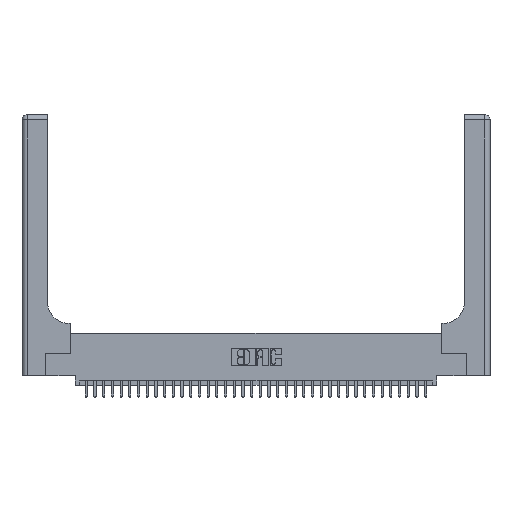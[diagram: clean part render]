
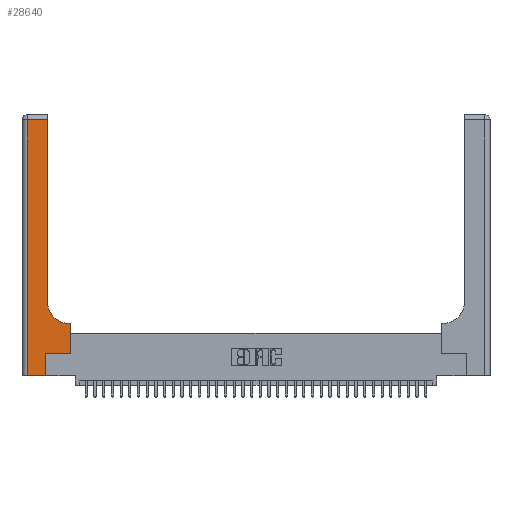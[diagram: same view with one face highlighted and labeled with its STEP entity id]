
A CAD part, top view. The second image highlights one B-rep face of the part: STEP entity #28640.
In plain terms, the highlighted planar face has unit normal (0, 0, 1).
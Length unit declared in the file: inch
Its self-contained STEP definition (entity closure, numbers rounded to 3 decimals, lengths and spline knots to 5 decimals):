
#216 = LINE ( 'NONE', #23032, #2450 ) ;
#758 = VERTEX_POINT ( 'NONE', #33562 ) ;
#1749 = ORIENTED_EDGE ( 'NONE', *, *, #3588, .T. ) ;
#1945 = FACE_OUTER_BOUND ( 'NONE', #30530, .T. ) ;
#2450 = VECTOR ( 'NONE', #5785, 39.37008 ) ;
#3264 = VERTEX_POINT ( 'NONE', #5364 ) ;
#3588 = EDGE_CURVE ( 'NONE', #25529, #7058, #6715, .T. ) ;
#4410 = VERTEX_POINT ( 'NONE', #25109 ) ;
#4511 = CARTESIAN_POINT ( 'NONE',  ( 0.269, 0.25, 0.37 ) ) ;
#5068 = VECTOR ( 'NONE', #15539, 39.37008 ) ;
#5190 = EDGE_CURVE ( 'NONE', #35783, #10188, #32566, .T. ) ;
#5364 = CARTESIAN_POINT ( 'NONE',  ( 0.269, 0., 0.37 ) ) ;
#5785 = DIRECTION ( 'NONE',  ( 1., 0., 0. ) ) ;
#5846 = EDGE_CURVE ( 'NONE', #9022, #7804, #28762, .T. ) ;
#6283 = ORIENTED_EDGE ( 'NONE', *, *, #30491, .T. ) ;
#6715 = LINE ( 'NONE', #29115, #36291 ) ;
#6791 = CARTESIAN_POINT ( 'NONE',  ( 0.269, 0.25, 0.37 ) ) ;
#7058 = VERTEX_POINT ( 'NONE', #10721 ) ;
#7113 = VECTOR ( 'NONE', #29776, 39.37008 ) ;
#7571 = CARTESIAN_POINT ( 'NONE',  ( 0., 2.94, 0.37 ) ) ;
#7800 = AXIS2_PLACEMENT_3D ( 'NONE', #9608, #24329, #23945 ) ;
#7804 = VERTEX_POINT ( 'NONE', #24131 ) ;
#9022 = VERTEX_POINT ( 'NONE', #18259 ) ;
#9608 = CARTESIAN_POINT ( 'NONE',  ( 0., 3., 0.37 ) ) ;
#10014 = EDGE_CURVE ( 'NONE', #3264, #35783, #19999, .T. ) ;
#10188 = VERTEX_POINT ( 'NONE', #33978 ) ;
#10332 = LINE ( 'NONE', #33193, #27759 ) ;
#10721 = CARTESIAN_POINT ( 'NONE',  ( 0.5415, 0.6, 0.37 ) ) ;
#11139 = EDGE_CURVE ( 'NONE', #4410, #758, #21702, .T. ) ;
#12292 = ORIENTED_EDGE ( 'NONE', *, *, #11139, .T. ) ;
#12838 = PLANE ( 'NONE',  #7800 ) ;
#14481 = ORIENTED_EDGE ( 'NONE', *, *, #5190, .T. ) ;
#15092 = CARTESIAN_POINT ( 'NONE',  ( 0.5585, 0.6, 0.37 ) ) ;
#15539 = DIRECTION ( 'NONE',  ( 0., -1., 0. ) ) ;
#17725 = ORIENTED_EDGE ( 'NONE', *, *, #23316, .T. ) ;
#18238 = VECTOR ( 'NONE', #27663, 39.37008 ) ;
#18259 = CARTESIAN_POINT ( 'NONE',  ( 0.06, 2.94, 0.37 ) ) ;
#18421 = DIRECTION ( 'NONE',  ( 0., 1., 0. ) ) ;
#18552 = CARTESIAN_POINT ( 'NONE',  ( 0.2915, 3., 0.37 ) ) ;
#18742 = LINE ( 'NONE', #7571, #18238 ) ;
#19999 = LINE ( 'NONE', #23917, #20849 ) ;
#20849 = VECTOR ( 'NONE', #32528, 39.37008 ) ;
#21106 = ORIENTED_EDGE ( 'NONE', *, *, #36372, .T. ) ;
#21702 = LINE ( 'NONE', #18552, #32864 ) ;
#21939 = ORIENTED_EDGE ( 'NONE', *, *, #25347, .T. ) ;
#22949 = CARTESIAN_POINT ( 'NONE',  ( 0.5415, 0.85, 0.37 ) ) ;
#23032 = CARTESIAN_POINT ( 'NONE',  ( 0., 0., 0.37 ) ) ;
#23316 = EDGE_CURVE ( 'NONE', #10188, #25529, #10332, .T. ) ;
#23917 = CARTESIAN_POINT ( 'NONE',  ( 0.269, 0., 0.37 ) ) ;
#23945 = DIRECTION ( 'NONE',  ( -1., 0., 0. ) ) ;
#24131 = CARTESIAN_POINT ( 'NONE',  ( 0.06, 0., 0.37 ) ) ;
#24329 = DIRECTION ( 'NONE',  ( 0., 0., -1. ) ) ;
#24713 = DIRECTION ( 'NONE',  ( 0., 1., 0. ) ) ;
#25109 = CARTESIAN_POINT ( 'NONE',  ( 0.2915, 0.85, 0.37 ) ) ;
#25347 = EDGE_CURVE ( 'NONE', #758, #9022, #18742, .T. ) ;
#25529 = VERTEX_POINT ( 'NONE', #15092 ) ;
#26757 = CIRCLE ( 'NONE', #36050, 0.25 ) ;
#26853 = DIRECTION ( 'NONE',  ( -1., 0., 0. ) ) ;
#27663 = DIRECTION ( 'NONE',  ( -1., 0., 0. ) ) ;
#27759 = VECTOR ( 'NONE', #24713, 39.37008 ) ;
#28591 = DIRECTION ( 'NONE',  ( 0., 0., -1. ) ) ;
#28640 = ADVANCED_FACE ( 'NONE', ( #1945 ), #12838, .F. ) ;
#28762 = LINE ( 'NONE', #32642, #5068 ) ;
#29115 = CARTESIAN_POINT ( 'NONE',  ( 0.2915, 0.6, 0.37 ) ) ;
#29776 = DIRECTION ( 'NONE',  ( 1., 0., 0. ) ) ;
#30302 = ORIENTED_EDGE ( 'NONE', *, *, #10014, .T. ) ;
#30491 = EDGE_CURVE ( 'NONE', #7058, #4410, #26757, .T. ) ;
#30530 = EDGE_LOOP ( 'NONE', ( #12292, #21939, #34489, #21106, #30302, #14481, #17725, #1749, #6283 ) ) ;
#31099 = DIRECTION ( 'NONE',  ( 1., 0., 0. ) ) ;
#32528 = DIRECTION ( 'NONE',  ( 0., 1., 0. ) ) ;
#32566 = LINE ( 'NONE', #6791, #7113 ) ;
#32642 = CARTESIAN_POINT ( 'NONE',  ( 0.06, 3., 0.37 ) ) ;
#32864 = VECTOR ( 'NONE', #18421, 39.37008 ) ;
#33193 = CARTESIAN_POINT ( 'NONE',  ( 0.5585, 0.25, 0.37 ) ) ;
#33562 = CARTESIAN_POINT ( 'NONE',  ( 0.2915, 2.94, 0.37 ) ) ;
#33978 = CARTESIAN_POINT ( 'NONE',  ( 0.5585, 0.25, 0.37 ) ) ;
#34489 = ORIENTED_EDGE ( 'NONE', *, *, #5846, .T. ) ;
#35783 = VERTEX_POINT ( 'NONE', #4511 ) ;
#36050 = AXIS2_PLACEMENT_3D ( 'NONE', #22949, #28591, #31099 ) ;
#36291 = VECTOR ( 'NONE', #26853, 39.37008 ) ;
#36372 = EDGE_CURVE ( 'NONE', #7804, #3264, #216, .T. ) ;
